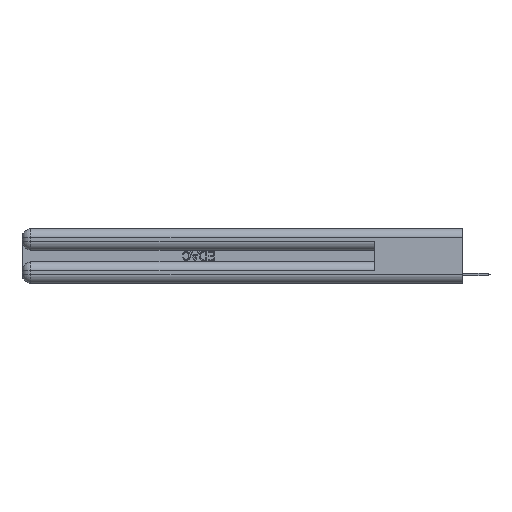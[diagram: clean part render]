
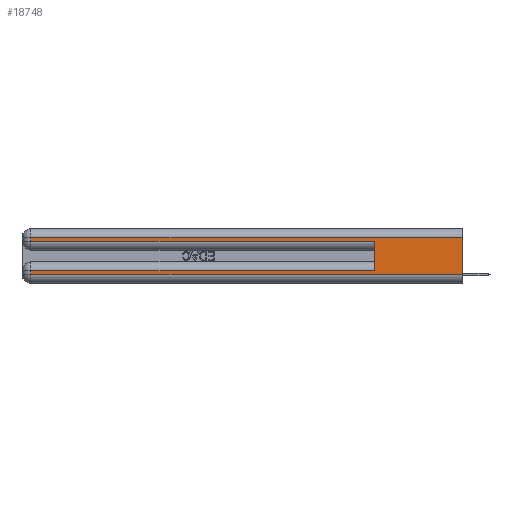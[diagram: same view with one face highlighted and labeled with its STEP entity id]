
A CAD part, left-side view. The second image highlights one B-rep face of the part: STEP entity #18748.
In plain terms, the highlighted planar face has unit normal (-1, 0, 0).
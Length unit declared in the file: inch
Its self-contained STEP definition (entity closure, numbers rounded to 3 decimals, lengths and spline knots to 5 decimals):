
#276 = LINE ( 'NONE', #26983, #6857 ) ;
#970 = LINE ( 'NONE', #22399, #17398 ) ;
#1322 = VERTEX_POINT ( 'NONE', #33860 ) ;
#2289 = CARTESIAN_POINT ( 'NONE',  ( 0., 0., 0.37 ) ) ;
#2438 = ORIENTED_EDGE ( 'NONE', *, *, #32269, .T. ) ;
#2486 = LINE ( 'NONE', #9700, #18137 ) ;
#2491 = ORIENTED_EDGE ( 'NONE', *, *, #12787, .F. ) ;
#3299 = VERTEX_POINT ( 'NONE', #12355 ) ;
#3687 = ORIENTED_EDGE ( 'NONE', *, *, #33986, .T. ) ;
#4840 = VERTEX_POINT ( 'NONE', #14254 ) ;
#4924 = DIRECTION ( 'NONE',  ( 0., 0., -1. ) ) ;
#5710 = ORIENTED_EDGE ( 'NONE', *, *, #11651, .T. ) ;
#5978 = VERTEX_POINT ( 'NONE', #23352 ) ;
#6857 = VECTOR ( 'NONE', #21704, 39.37008 ) ;
#7062 = DIRECTION ( 'NONE',  ( 0., 0., -1. ) ) ;
#7279 = VERTEX_POINT ( 'NONE', #7888 ) ;
#7475 = ORIENTED_EDGE ( 'NONE', *, *, #31707, .T. ) ;
#7888 = CARTESIAN_POINT ( 'NONE',  ( 0., 0.6, 0.085 ) ) ;
#8046 = CARTESIAN_POINT ( 'NONE',  ( 0., 2.94, 0.285 ) ) ;
#8407 = CARTESIAN_POINT ( 'NONE',  ( 0., 0.6, 0.145 ) ) ;
#8839 = CARTESIAN_POINT ( 'NONE',  ( 0., 0., 0.06 ) ) ;
#9451 = EDGE_CURVE ( 'NONE', #14986, #5978, #31973, .T. ) ;
#9700 = CARTESIAN_POINT ( 'NONE',  ( 0., 2.94, 0.37 ) ) ;
#10193 = FACE_OUTER_BOUND ( 'NONE', #26354, .T. ) ;
#11651 = EDGE_CURVE ( 'NONE', #7279, #3299, #970, .T. ) ;
#12355 = CARTESIAN_POINT ( 'NONE',  ( 0., 2.94, 0.085 ) ) ;
#12688 = VERTEX_POINT ( 'NONE', #20542 ) ;
#12787 = EDGE_CURVE ( 'NONE', #7279, #1322, #30014, .T. ) ;
#12807 = VECTOR ( 'NONE', #15988, 39.37008 ) ;
#13059 = VECTOR ( 'NONE', #25003, 39.37008 ) ;
#13310 = DIRECTION ( 'NONE',  ( 0., 0., -1. ) ) ;
#13523 = CARTESIAN_POINT ( 'NONE',  ( 0., 0., 0.31 ) ) ;
#13587 = ORIENTED_EDGE ( 'NONE', *, *, #9451, .T. ) ;
#14254 = CARTESIAN_POINT ( 'NONE',  ( 0., 2.94, 0.06 ) ) ;
#14986 = VERTEX_POINT ( 'NONE', #16783 ) ;
#15121 = PLANE ( 'NONE',  #29266 ) ;
#15988 = DIRECTION ( 'NONE',  ( 0., 1., 0. ) ) ;
#16521 = VECTOR ( 'NONE', #20236, 39.37008 ) ;
#16783 = CARTESIAN_POINT ( 'NONE',  ( 0., 0., 0.31 ) ) ;
#17398 = VECTOR ( 'NONE', #27850, 39.37008 ) ;
#17429 = LINE ( 'NONE', #20577, #16521 ) ;
#18137 = VECTOR ( 'NONE', #7062, 39.37008 ) ;
#18178 = VECTOR ( 'NONE', #13310, 39.37008 ) ;
#18748 = ADVANCED_FACE ( 'NONE', ( #10193 ), #15121, .F. ) ;
#19464 = ORIENTED_EDGE ( 'NONE', *, *, #32392, .T. ) ;
#20236 = DIRECTION ( 'NONE',  ( 0., 0., -1. ) ) ;
#20542 = CARTESIAN_POINT ( 'NONE',  ( 0., 0., 0.06 ) ) ;
#20577 = CARTESIAN_POINT ( 'NONE',  ( 0., 2.94, 0.37 ) ) ;
#20728 = DIRECTION ( 'NONE',  ( 1., 0., 0. ) ) ;
#21704 = DIRECTION ( 'NONE',  ( 0., -1., 0. ) ) ;
#21922 = DIRECTION ( 'NONE',  ( 0., 0., 1. ) ) ;
#22399 = CARTESIAN_POINT ( 'NONE',  ( 0., 0., 0.085 ) ) ;
#23211 = EDGE_CURVE ( 'NONE', #14986, #12688, #26674, .T. ) ;
#23352 = CARTESIAN_POINT ( 'NONE',  ( 0., 2.94, 0.31 ) ) ;
#25003 = DIRECTION ( 'NONE',  ( 0., -1., 0. ) ) ;
#25937 = VERTEX_POINT ( 'NONE', #8046 ) ;
#26354 = EDGE_LOOP ( 'NONE', ( #29739, #13587, #3687, #7475, #2491, #5710, #19464, #2438 ) ) ;
#26674 = LINE ( 'NONE', #27022, #18178 ) ;
#26983 = CARTESIAN_POINT ( 'NONE',  ( 0., 0., 0.285 ) ) ;
#27022 = CARTESIAN_POINT ( 'NONE',  ( 0., 0., 0.37 ) ) ;
#27814 = LINE ( 'NONE', #8839, #13059 ) ;
#27850 = DIRECTION ( 'NONE',  ( 0., 1., 0. ) ) ;
#29266 = AXIS2_PLACEMENT_3D ( 'NONE', #2289, #20728, #4924 ) ;
#29739 = ORIENTED_EDGE ( 'NONE', *, *, #23211, .F. ) ;
#30014 = LINE ( 'NONE', #8407, #30926 ) ;
#30926 = VECTOR ( 'NONE', #21922, 39.37008 ) ;
#31707 = EDGE_CURVE ( 'NONE', #25937, #1322, #276, .T. ) ;
#31973 = LINE ( 'NONE', #13523, #12807 ) ;
#32269 = EDGE_CURVE ( 'NONE', #4840, #12688, #27814, .T. ) ;
#32392 = EDGE_CURVE ( 'NONE', #3299, #4840, #2486, .T. ) ;
#33860 = CARTESIAN_POINT ( 'NONE',  ( 0., 0.6, 0.285 ) ) ;
#33986 = EDGE_CURVE ( 'NONE', #5978, #25937, #17429, .T. ) ;
